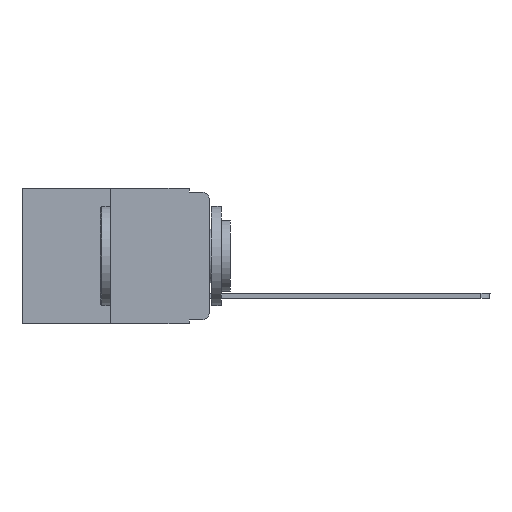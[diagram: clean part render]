
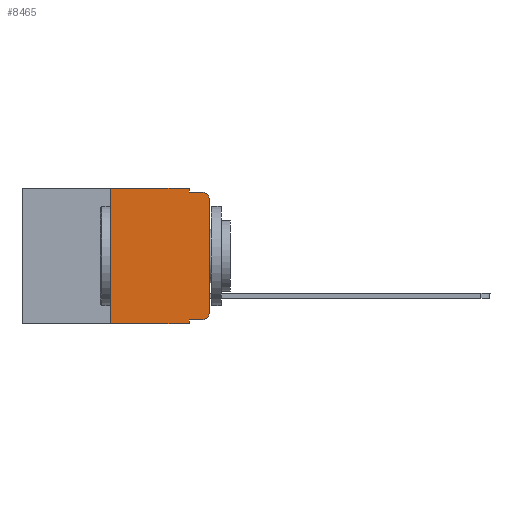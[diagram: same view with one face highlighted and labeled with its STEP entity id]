
A CAD part, left-side view. The second image highlights one B-rep face of the part: STEP entity #8465.
In plain terms, the highlighted planar face has unit normal (-1, 0, 0).
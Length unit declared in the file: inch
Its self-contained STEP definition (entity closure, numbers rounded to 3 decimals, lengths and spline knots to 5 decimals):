
#65 = AXIS2_PLACEMENT_3D ( 'NONE', #10632, #11392, #3961 ) ;
#80 = LINE ( 'NONE', #2726, #11060 ) ;
#358 = PLANE ( 'NONE',  #4011 ) ;
#424 = EDGE_CURVE ( 'NONE', #5254, #2624, #6143, .T. ) ;
#480 = CARTESIAN_POINT ( 'NONE',  ( 0., 0.051, -0.01 ) ) ;
#494 = CARTESIAN_POINT ( 'NONE',  ( 0., 0., 0. ) ) ;
#502 = DIRECTION ( 'NONE',  ( 0., 0., 1. ) ) ;
#533 = LINE ( 'NONE', #3651, #8559 ) ;
#1093 = CARTESIAN_POINT ( 'NONE',  ( 0., 0.25, -0.343 ) ) ;
#1323 = ORIENTED_EDGE ( 'NONE', *, *, #2136, .F. ) ;
#2051 = ORIENTED_EDGE ( 'NONE', *, *, #8406, .T. ) ;
#2097 = CARTESIAN_POINT ( 'NONE',  ( 0., 0.051, 0. ) ) ;
#2136 = EDGE_CURVE ( 'NONE', #5627, #5379, #7602, .T. ) ;
#2311 = VECTOR ( 'NONE', #11639, 39.37008 ) ;
#2391 = CARTESIAN_POINT ( 'NONE',  ( 0., 0., -0.313 ) ) ;
#2624 = VERTEX_POINT ( 'NONE', #5025 ) ;
#2726 = CARTESIAN_POINT ( 'NONE',  ( 0., 0.473, 0. ) ) ;
#2826 = LINE ( 'NONE', #5626, #10874 ) ;
#2903 = LINE ( 'NONE', #10926, #5080 ) ;
#3052 = ORIENTED_EDGE ( 'NONE', *, *, #7015, .F. ) ;
#3312 = CARTESIAN_POINT ( 'NONE',  ( 0., 0.051, -0.343 ) ) ;
#3376 = CIRCLE ( 'NONE', #9757, 0.02 ) ;
#3429 = VERTEX_POINT ( 'NONE', #4009 ) ;
#3459 = VECTOR ( 'NONE', #4701, 39.37008 ) ;
#3651 = CARTESIAN_POINT ( 'NONE',  ( 0., 0.051, 0. ) ) ;
#3758 = DIRECTION ( 'NONE',  ( 0., -1., 0. ) ) ;
#3774 = ORIENTED_EDGE ( 'NONE', *, *, #424, .F. ) ;
#3852 = FACE_OUTER_BOUND ( 'NONE', #9335, .T. ) ;
#3854 = CARTESIAN_POINT ( 'NONE',  ( 0., 0.473, -0.343 ) ) ;
#3880 = ORIENTED_EDGE ( 'NONE', *, *, #6526, .F. ) ;
#3885 = CARTESIAN_POINT ( 'NONE',  ( 0., 0., -0.03 ) ) ;
#3961 = DIRECTION ( 'NONE',  ( 0., 0., -1. ) ) ;
#4009 = CARTESIAN_POINT ( 'NONE',  ( 0., 0.051, -0.333 ) ) ;
#4011 = AXIS2_PLACEMENT_3D ( 'NONE', #11598, #4024, #7730 ) ;
#4024 = DIRECTION ( 'NONE',  ( 1., 0., 0. ) ) ;
#4196 = EDGE_CURVE ( 'NONE', #5072, #7478, #9074, .T. ) ;
#4300 = DIRECTION ( 'NONE',  ( 0., 0., -1. ) ) ;
#4623 = LINE ( 'NONE', #3854, #3459 ) ;
#4701 = DIRECTION ( 'NONE',  ( 0., -1., 0. ) ) ;
#4707 = VECTOR ( 'NONE', #502, 39.37008 ) ;
#4843 = DIRECTION ( 'NONE',  ( 0., -1., 0. ) ) ;
#5025 = CARTESIAN_POINT ( 'NONE',  ( 0., 0.25, 0. ) ) ;
#5072 = VERTEX_POINT ( 'NONE', #7377 ) ;
#5080 = VECTOR ( 'NONE', #4300, 39.37008 ) ;
#5186 = DIRECTION ( 'NONE',  ( 0., -1., 0. ) ) ;
#5254 = VERTEX_POINT ( 'NONE', #1093 ) ;
#5379 = VERTEX_POINT ( 'NONE', #11434 ) ;
#5626 = CARTESIAN_POINT ( 'NONE',  ( 0., 0.051, -0.333 ) ) ;
#5627 = VERTEX_POINT ( 'NONE', #6280 ) ;
#5884 = EDGE_CURVE ( 'NONE', #5254, #11017, #4623, .T. ) ;
#5940 = VERTEX_POINT ( 'NONE', #2097 ) ;
#5989 = ORIENTED_EDGE ( 'NONE', *, *, #10047, .T. ) ;
#6143 = LINE ( 'NONE', #11412, #4707 ) ;
#6280 = CARTESIAN_POINT ( 'NONE',  ( 0., 0.051, -0.01 ) ) ;
#6458 = CARTESIAN_POINT ( 'NONE',  ( 0., 0.02, -0.03 ) ) ;
#6489 = DIRECTION ( 'NONE',  ( -1., 0., 0. ) ) ;
#6526 = EDGE_CURVE ( 'NONE', #5940, #5627, #533, .T. ) ;
#7015 = EDGE_CURVE ( 'NONE', #2624, #5940, #80, .T. ) ;
#7377 = CARTESIAN_POINT ( 'NONE',  ( 0., 0.02, -0.333 ) ) ;
#7478 = VERTEX_POINT ( 'NONE', #2391 ) ;
#7602 = LINE ( 'NONE', #480, #11405 ) ;
#7730 = DIRECTION ( 'NONE',  ( 0., 0., -1. ) ) ;
#7831 = ORIENTED_EDGE ( 'NONE', *, *, #11083, .F. ) ;
#8301 = DIRECTION ( 'NONE',  ( 0., 0., -1. ) ) ;
#8406 = EDGE_CURVE ( 'NONE', #3429, #5072, #2826, .T. ) ;
#8465 = ADVANCED_FACE ( 'NONE', ( #3852 ), #358, .F. ) ;
#8559 = VECTOR ( 'NONE', #11192, 39.37008 ) ;
#9074 = CIRCLE ( 'NONE', #65, 0.02 ) ;
#9081 = VERTEX_POINT ( 'NONE', #3885 ) ;
#9335 = EDGE_LOOP ( 'NONE', ( #11074, #5989, #1323, #3880, #3052, #3774, #10460, #7831, #2051, #10209 ) ) ;
#9757 = AXIS2_PLACEMENT_3D ( 'NONE', #6458, #6489, #8301 ) ;
#10047 = EDGE_CURVE ( 'NONE', #9081, #5379, #3376, .T. ) ;
#10209 = ORIENTED_EDGE ( 'NONE', *, *, #4196, .T. ) ;
#10460 = ORIENTED_EDGE ( 'NONE', *, *, #5884, .T. ) ;
#10632 = CARTESIAN_POINT ( 'NONE',  ( 0., 0.02, -0.313 ) ) ;
#10874 = VECTOR ( 'NONE', #4843, 39.37008 ) ;
#10926 = CARTESIAN_POINT ( 'NONE',  ( 0., 0.051, 0. ) ) ;
#11017 = VERTEX_POINT ( 'NONE', #3312 ) ;
#11060 = VECTOR ( 'NONE', #3758, 39.37008 ) ;
#11074 = ORIENTED_EDGE ( 'NONE', *, *, #11629, .T. ) ;
#11083 = EDGE_CURVE ( 'NONE', #3429, #11017, #2903, .T. ) ;
#11192 = DIRECTION ( 'NONE',  ( 0., 0., -1. ) ) ;
#11392 = DIRECTION ( 'NONE',  ( -1., 0., 0. ) ) ;
#11405 = VECTOR ( 'NONE', #5186, 39.37008 ) ;
#11412 = CARTESIAN_POINT ( 'NONE',  ( 0., 0.25, 0. ) ) ;
#11434 = CARTESIAN_POINT ( 'NONE',  ( 0., 0.02, -0.01 ) ) ;
#11598 = CARTESIAN_POINT ( 'NONE',  ( 0., 0.473, 0. ) ) ;
#11629 = EDGE_CURVE ( 'NONE', #7478, #9081, #12085, .T. ) ;
#11639 = DIRECTION ( 'NONE',  ( 0., 0., 1. ) ) ;
#12085 = LINE ( 'NONE', #494, #2311 ) ;
